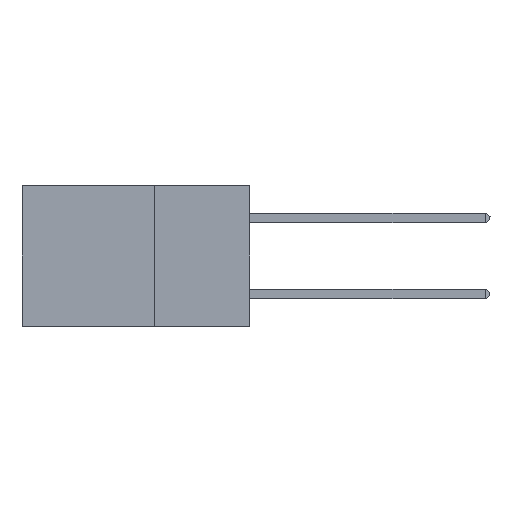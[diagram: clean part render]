
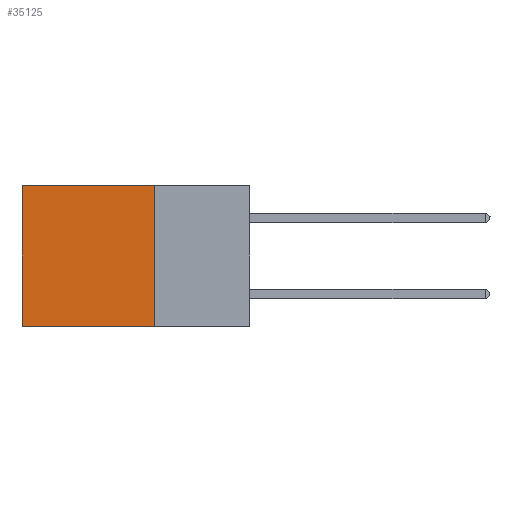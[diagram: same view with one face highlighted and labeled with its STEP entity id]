
A CAD part, left-side view. The second image highlights one B-rep face of the part: STEP entity #35125.
In plain terms, the highlighted planar face has unit normal (-1, 0, 0).
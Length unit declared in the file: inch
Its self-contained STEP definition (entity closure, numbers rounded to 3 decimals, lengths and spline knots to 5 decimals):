
#792 = CARTESIAN_POINT ( 'NONE',  ( 0.2875, 0.6, -0.37 ) ) ;
#1349 = VECTOR ( 'NONE', #2224, 39.37008 ) ;
#1361 = EDGE_CURVE ( 'NONE', #2194, #31523, #37250, .T. ) ;
#1848 = EDGE_LOOP ( 'NONE', ( #30544, #33403, #20892, #19589 ) ) ;
#2194 = VERTEX_POINT ( 'NONE', #20479 ) ;
#2212 = LINE ( 'NONE', #31633, #12275 ) ;
#2224 = DIRECTION ( 'NONE',  ( 0., 1., 0. ) ) ;
#3347 = AXIS2_PLACEMENT_3D ( 'NONE', #25076, #4013, #12373 ) ;
#4013 = DIRECTION ( 'NONE',  ( 1., 0., 0. ) ) ;
#5013 = CARTESIAN_POINT ( 'NONE',  ( 0.2875, 0.25, 0. ) ) ;
#6657 = CARTESIAN_POINT ( 'NONE',  ( 0.2875, 0.25, -0.37 ) ) ;
#8268 = LINE ( 'NONE', #11044, #17761 ) ;
#9267 = CARTESIAN_POINT ( 'NONE',  ( 0.2875, 0.25, 0. ) ) ;
#11044 = CARTESIAN_POINT ( 'NONE',  ( 0.2875, 0.6, 0. ) ) ;
#12175 = VERTEX_POINT ( 'NONE', #31296 ) ;
#12275 = VECTOR ( 'NONE', #17313, 39.37008 ) ;
#12373 = DIRECTION ( 'NONE',  ( 0., 0., -1. ) ) ;
#15549 = PLANE ( 'NONE',  #3347 ) ;
#17054 = VECTOR ( 'NONE', #24939, 39.37008 ) ;
#17313 = DIRECTION ( 'NONE',  ( 0., 0., -1. ) ) ;
#17761 = VECTOR ( 'NONE', #26346, 39.37008 ) ;
#19589 = ORIENTED_EDGE ( 'NONE', *, *, #33800, .T. ) ;
#20262 = VERTEX_POINT ( 'NONE', #9267 ) ;
#20479 = CARTESIAN_POINT ( 'NONE',  ( 0.2875, 0.25, -0.37 ) ) ;
#20892 = ORIENTED_EDGE ( 'NONE', *, *, #36583, .F. ) ;
#22287 = FACE_OUTER_BOUND ( 'NONE', #1848, .T. ) ;
#24939 = DIRECTION ( 'NONE',  ( 0., 1., 0. ) ) ;
#25076 = CARTESIAN_POINT ( 'NONE',  ( 0.2875, 0.25, 0. ) ) ;
#26346 = DIRECTION ( 'NONE',  ( 0., 0., -1. ) ) ;
#30269 = EDGE_CURVE ( 'NONE', #12175, #31523, #8268, .T. ) ;
#30544 = ORIENTED_EDGE ( 'NONE', *, *, #30269, .T. ) ;
#31296 = CARTESIAN_POINT ( 'NONE',  ( 0.2875, 0.6, 0. ) ) ;
#31523 = VERTEX_POINT ( 'NONE', #792 ) ;
#31633 = CARTESIAN_POINT ( 'NONE',  ( 0.2875, 0.25, 0. ) ) ;
#32225 = LINE ( 'NONE', #5013, #1349 ) ;
#33403 = ORIENTED_EDGE ( 'NONE', *, *, #1361, .F. ) ;
#33800 = EDGE_CURVE ( 'NONE', #20262, #12175, #32225, .T. ) ;
#35125 = ADVANCED_FACE ( 'NONE', ( #22287 ), #15549, .F. ) ;
#36583 = EDGE_CURVE ( 'NONE', #20262, #2194, #2212, .T. ) ;
#37250 = LINE ( 'NONE', #6657, #17054 ) ;
